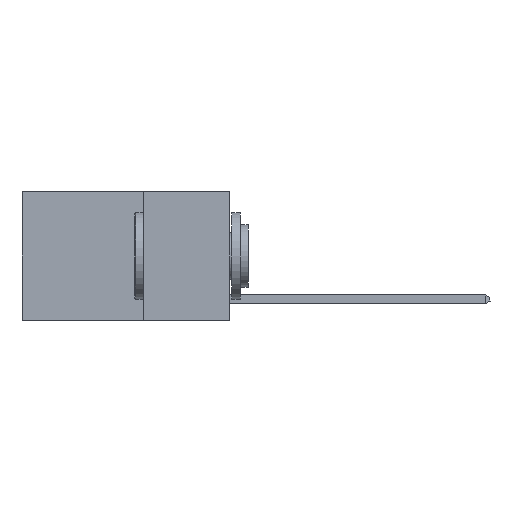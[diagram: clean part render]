
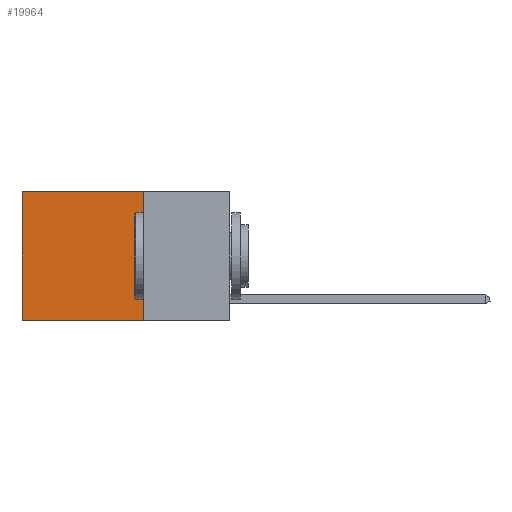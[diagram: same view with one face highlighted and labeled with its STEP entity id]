
A CAD part, left-side view. The second image highlights one B-rep face of the part: STEP entity #19964.
In plain terms, the highlighted planar face has unit normal (-1, 0, 0).
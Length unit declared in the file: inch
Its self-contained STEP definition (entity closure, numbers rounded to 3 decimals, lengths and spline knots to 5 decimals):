
#1296 = VERTEX_POINT ( 'NONE', #14985 ) ;
#1576 = DIRECTION ( 'NONE',  ( 0., 0., -1. ) ) ;
#2776 = CARTESIAN_POINT ( 'NONE',  ( 0.2625, 0.25, 0. ) ) ;
#2968 = EDGE_LOOP ( 'NONE', ( #18156, #4800, #6803, #14189 ) ) ;
#3628 = CARTESIAN_POINT ( 'NONE',  ( 0.2625, 0.25, 0. ) ) ;
#4088 = DIRECTION ( 'NONE',  ( 1., 0., 0. ) ) ;
#4310 = CARTESIAN_POINT ( 'NONE',  ( 0.2625, 0.6, 0. ) ) ;
#4800 = ORIENTED_EDGE ( 'NONE', *, *, #13795, .F. ) ;
#5442 = DIRECTION ( 'NONE',  ( 0., 1., 0. ) ) ;
#6461 = EDGE_CURVE ( 'NONE', #20232, #6875, #16032, .T. ) ;
#6722 = VECTOR ( 'NONE', #11654, 39.37008 ) ;
#6803 = ORIENTED_EDGE ( 'NONE', *, *, #18177, .F. ) ;
#6875 = VERTEX_POINT ( 'NONE', #4310 ) ;
#7352 = CARTESIAN_POINT ( 'NONE',  ( 0.2625, 0.25, 0. ) ) ;
#7917 = VECTOR ( 'NONE', #1576, 39.37008 ) ;
#8448 = LINE ( 'NONE', #11543, #6722 ) ;
#8543 = LINE ( 'NONE', #10299, #15157 ) ;
#9455 = VERTEX_POINT ( 'NONE', #20857 ) ;
#9940 = EDGE_CURVE ( 'NONE', #6875, #9455, #8448, .T. ) ;
#9942 = LINE ( 'NONE', #16702, #7917 ) ;
#10299 = CARTESIAN_POINT ( 'NONE',  ( 0.2625, 0.25, -0.37 ) ) ;
#10846 = VECTOR ( 'NONE', #19267, 39.37008 ) ;
#11543 = CARTESIAN_POINT ( 'NONE',  ( 0.2625, 0.6, 0. ) ) ;
#11654 = DIRECTION ( 'NONE',  ( 0., 0., -1. ) ) ;
#12226 = PLANE ( 'NONE',  #18032 ) ;
#13795 = EDGE_CURVE ( 'NONE', #1296, #9455, #8543, .T. ) ;
#13994 = DIRECTION ( 'NONE',  ( 0., 0., -1. ) ) ;
#14189 = ORIENTED_EDGE ( 'NONE', *, *, #6461, .T. ) ;
#14985 = CARTESIAN_POINT ( 'NONE',  ( 0.2625, 0.25, -0.37 ) ) ;
#15157 = VECTOR ( 'NONE', #5442, 39.37008 ) ;
#16032 = LINE ( 'NONE', #2776, #10846 ) ;
#16702 = CARTESIAN_POINT ( 'NONE',  ( 0.2625, 0.25, 0. ) ) ;
#17661 = FACE_OUTER_BOUND ( 'NONE', #2968, .T. ) ;
#18032 = AXIS2_PLACEMENT_3D ( 'NONE', #7352, #4088, #13994 ) ;
#18156 = ORIENTED_EDGE ( 'NONE', *, *, #9940, .T. ) ;
#18177 = EDGE_CURVE ( 'NONE', #20232, #1296, #9942, .T. ) ;
#19267 = DIRECTION ( 'NONE',  ( 0., 1., 0. ) ) ;
#19964 = ADVANCED_FACE ( 'NONE', ( #17661 ), #12226, .F. ) ;
#20232 = VERTEX_POINT ( 'NONE', #3628 ) ;
#20857 = CARTESIAN_POINT ( 'NONE',  ( 0.2625, 0.6, -0.37 ) ) ;
